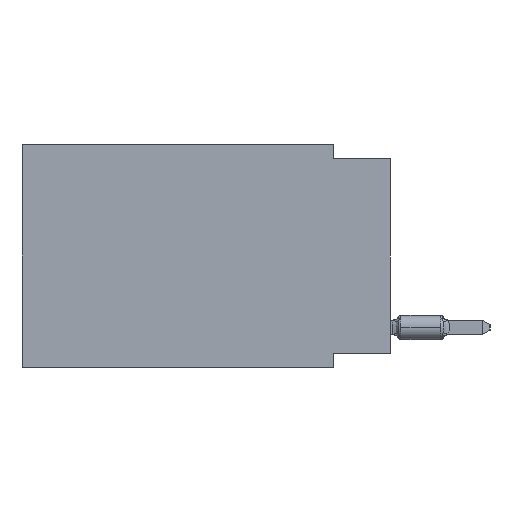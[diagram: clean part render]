
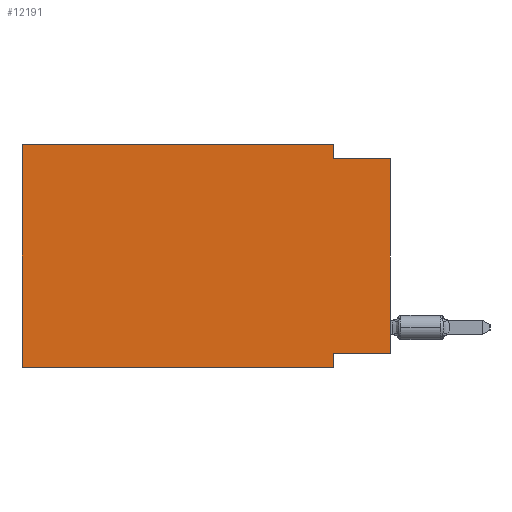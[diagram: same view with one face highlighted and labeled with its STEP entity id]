
A CAD part, left-side view. The second image highlights one B-rep face of the part: STEP entity #12191.
In plain terms, the highlighted planar face has unit normal (-1, 0, 0).
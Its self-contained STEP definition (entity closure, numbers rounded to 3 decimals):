
#60 = VECTOR ( 'NONE', #7682, 1000. ) ;
#949 = LINE ( 'NONE', #20922, #20177 ) ;
#1586 = LINE ( 'NONE', #28498, #42252 ) ;
#1755 = CARTESIAN_POINT ( 'NONE',  ( 0., 2.54, 0. ) ) ;
#4611 = VERTEX_POINT ( 'NONE', #40252 ) ;
#7363 = VECTOR ( 'NONE', #25012, 1000. ) ;
#7425 = LINE ( 'NONE', #21091, #35997 ) ;
#7682 = DIRECTION ( 'NONE',  ( 0., -1., 0. ) ) ;
#8013 = ORIENTED_EDGE ( 'NONE', *, *, #8211, .T. ) ;
#8211 = EDGE_CURVE ( 'NONE', #9895, #36828, #949, .T. ) ;
#9368 = ORIENTED_EDGE ( 'NONE', *, *, #38347, .F. ) ;
#9483 = CARTESIAN_POINT ( 'NONE',  ( 0., 16.383, 0. ) ) ;
#9895 = VERTEX_POINT ( 'NONE', #36933 ) ;
#10704 = VECTOR ( 'NONE', #23129, 1000. ) ;
#10937 = DIRECTION ( 'NONE',  ( 0., 0., -1. ) ) ;
#11814 = CARTESIAN_POINT ( 'NONE',  ( 0., 16.383, -9.906 ) ) ;
#11866 = ORIENTED_EDGE ( 'NONE', *, *, #34388, .T. ) ;
#12191 = ADVANCED_FACE ( 'NONE', ( #20998 ), #20333, .F. ) ;
#12545 = EDGE_LOOP ( 'NONE', ( #8013, #9368, #21852, #40011, #12708, #11866, #28455, #40463 ) ) ;
#12708 = ORIENTED_EDGE ( 'NONE', *, *, #25434, .F. ) ;
#12743 = CARTESIAN_POINT ( 'NONE',  ( 0., 2.54, 0. ) ) ;
#13942 = CARTESIAN_POINT ( 'NONE',  ( 0., 2.54, -9.906 ) ) ;
#15047 = VERTEX_POINT ( 'NONE', #13942 ) ;
#16861 = AXIS2_PLACEMENT_3D ( 'NONE', #37347, #24354, #33983 ) ;
#16930 = CARTESIAN_POINT ( 'NONE',  ( 0., 2.54, -9.271 ) ) ;
#19086 = EDGE_CURVE ( 'NONE', #44110, #24553, #40143, .T. ) ;
#20177 = VECTOR ( 'NONE', #34574, 1000. ) ;
#20182 = VECTOR ( 'NONE', #26185, 1000. ) ;
#20333 = PLANE ( 'NONE',  #16861 ) ;
#20441 = VECTOR ( 'NONE', #10937, 1000. ) ;
#20922 = CARTESIAN_POINT ( 'NONE',  ( 0., 0., 0. ) ) ;
#20998 = FACE_OUTER_BOUND ( 'NONE', #12545, .T. ) ;
#21091 = CARTESIAN_POINT ( 'NONE',  ( 0., 0., -0.635 ) ) ;
#21122 = LINE ( 'NONE', #27408, #60 ) ;
#21852 = ORIENTED_EDGE ( 'NONE', *, *, #24573, .F. ) ;
#23129 = DIRECTION ( 'NONE',  ( 0., -1., 0. ) ) ;
#24354 = DIRECTION ( 'NONE',  ( 1., 0., 0. ) ) ;
#24553 = VERTEX_POINT ( 'NONE', #1755 ) ;
#24573 = EDGE_CURVE ( 'NONE', #24553, #4611, #36036, .T. ) ;
#24593 = CARTESIAN_POINT ( 'NONE',  ( 0., 2.54, -9.906 ) ) ;
#25012 = DIRECTION ( 'NONE',  ( 0., 0., 1. ) ) ;
#25434 = EDGE_CURVE ( 'NONE', #37276, #44110, #35096, .T. ) ;
#26185 = DIRECTION ( 'NONE',  ( 0., 0., -1. ) ) ;
#27408 = CARTESIAN_POINT ( 'NONE',  ( 0., 16.383, -9.906 ) ) ;
#27818 = DIRECTION ( 'NONE',  ( 0., -1., 0. ) ) ;
#28321 = EDGE_CURVE ( 'NONE', #41544, #15047, #35116, .T. ) ;
#28455 = ORIENTED_EDGE ( 'NONE', *, *, #28321, .F. ) ;
#28498 = CARTESIAN_POINT ( 'NONE',  ( 0., 0., -9.271 ) ) ;
#28609 = CARTESIAN_POINT ( 'NONE',  ( 0., 16.383, 0. ) ) ;
#32511 = DIRECTION ( 'NONE',  ( 0., 1., 0. ) ) ;
#33983 = DIRECTION ( 'NONE',  ( 0., 0., -1. ) ) ;
#34388 = EDGE_CURVE ( 'NONE', #37276, #15047, #21122, .T. ) ;
#34574 = DIRECTION ( 'NONE',  ( 0., 0., 1. ) ) ;
#35096 = LINE ( 'NONE', #28609, #7363 ) ;
#35116 = LINE ( 'NONE', #24593, #20441 ) ;
#35254 = EDGE_CURVE ( 'NONE', #9895, #41544, #1586, .T. ) ;
#35997 = VECTOR ( 'NONE', #27818, 1000. ) ;
#36036 = LINE ( 'NONE', #12743, #20182 ) ;
#36241 = CARTESIAN_POINT ( 'NONE',  ( 0., 16.383, 0. ) ) ;
#36828 = VERTEX_POINT ( 'NONE', #38737 ) ;
#36933 = CARTESIAN_POINT ( 'NONE',  ( 0., 0., -9.271 ) ) ;
#37276 = VERTEX_POINT ( 'NONE', #11814 ) ;
#37347 = CARTESIAN_POINT ( 'NONE',  ( 0., 16.383, 0. ) ) ;
#38347 = EDGE_CURVE ( 'NONE', #4611, #36828, #7425, .T. ) ;
#38737 = CARTESIAN_POINT ( 'NONE',  ( 0., 0., -0.635 ) ) ;
#40011 = ORIENTED_EDGE ( 'NONE', *, *, #19086, .F. ) ;
#40143 = LINE ( 'NONE', #9483, #10704 ) ;
#40252 = CARTESIAN_POINT ( 'NONE',  ( 0., 2.54, -0.635 ) ) ;
#40463 = ORIENTED_EDGE ( 'NONE', *, *, #35254, .F. ) ;
#41544 = VERTEX_POINT ( 'NONE', #16930 ) ;
#42252 = VECTOR ( 'NONE', #32511, 1000. ) ;
#44110 = VERTEX_POINT ( 'NONE', #36241 ) ;
